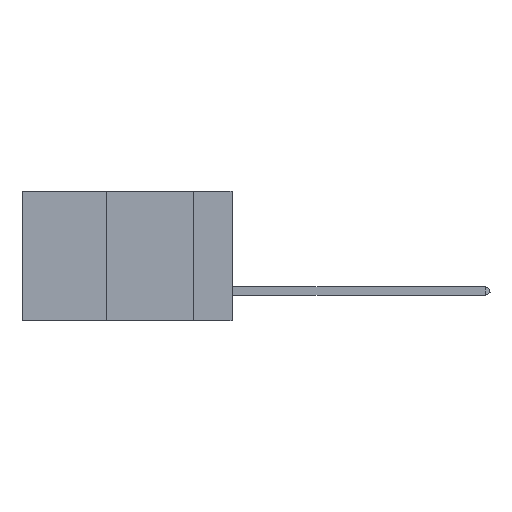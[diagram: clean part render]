
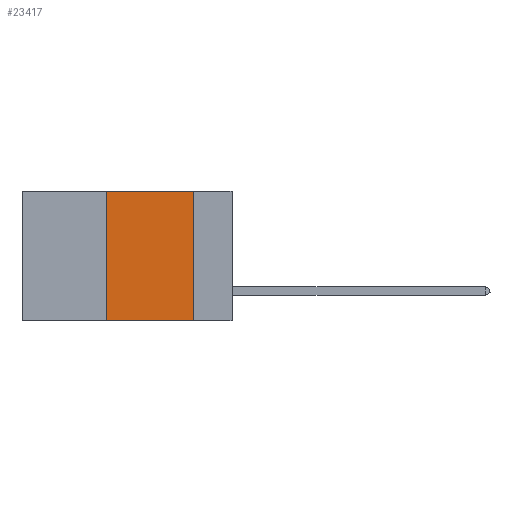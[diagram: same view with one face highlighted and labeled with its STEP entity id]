
A CAD part, left-side view. The second image highlights one B-rep face of the part: STEP entity #23417.
In plain terms, the highlighted planar face has unit normal (-1, 0, 0).
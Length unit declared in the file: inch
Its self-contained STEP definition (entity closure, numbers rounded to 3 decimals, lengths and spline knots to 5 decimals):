
#2882 = ORIENTED_EDGE ( 'NONE', *, *, #22673, .F. ) ;
#3246 = CARTESIAN_POINT ( 'NONE',  ( 0., 0.36, 0. ) ) ;
#4315 = LINE ( 'NONE', #11277, #26210 ) ;
#4737 = ORIENTED_EDGE ( 'NONE', *, *, #27943, .T. ) ;
#5513 = EDGE_CURVE ( 'NONE', #7161, #22218, #30814, .T. ) ;
#6093 = DIRECTION ( 'NONE',  ( 0., -1., 0. ) ) ;
#6734 = CARTESIAN_POINT ( 'NONE',  ( 0., 0.6, 0. ) ) ;
#7047 = ORIENTED_EDGE ( 'NONE', *, *, #29732, .F. ) ;
#7161 = VERTEX_POINT ( 'NONE', #10127 ) ;
#7401 = DIRECTION ( 'NONE',  ( 0., -1., 0. ) ) ;
#8808 = PLANE ( 'NONE',  #25609 ) ;
#10127 = CARTESIAN_POINT ( 'NONE',  ( 0., 0.36, 0. ) ) ;
#11152 = VECTOR ( 'NONE', #6093, 39.37008 ) ;
#11186 = VECTOR ( 'NONE', #7401, 39.37008 ) ;
#11277 = CARTESIAN_POINT ( 'NONE',  ( 0., 0.11, 0. ) ) ;
#11842 = VERTEX_POINT ( 'NONE', #31393 ) ;
#12524 = CARTESIAN_POINT ( 'NONE',  ( 0., 0.6, -0.37 ) ) ;
#14670 = CARTESIAN_POINT ( 'NONE',  ( 0., 0.11, -0.37 ) ) ;
#15734 = FACE_OUTER_BOUND ( 'NONE', #24932, .T. ) ;
#18116 = LINE ( 'NONE', #12524, #11186 ) ;
#20738 = DIRECTION ( 'NONE',  ( 1., 0., 0. ) ) ;
#20935 = DIRECTION ( 'NONE',  ( 0., 0., -1. ) ) ;
#21161 = CARTESIAN_POINT ( 'NONE',  ( 0., 0.6, 0. ) ) ;
#21853 = VERTEX_POINT ( 'NONE', #14670 ) ;
#22218 = VERTEX_POINT ( 'NONE', #28332 ) ;
#22450 = DIRECTION ( 'NONE',  ( 0., 0., 1. ) ) ;
#22673 = EDGE_CURVE ( 'NONE', #22218, #21853, #4315, .T. ) ;
#23417 = ADVANCED_FACE ( 'NONE', ( #15734 ), #8808, .F. ) ;
#24184 = ORIENTED_EDGE ( 'NONE', *, *, #5513, .F. ) ;
#24932 = EDGE_LOOP ( 'NONE', ( #2882, #24184, #7047, #4737 ) ) ;
#25609 = AXIS2_PLACEMENT_3D ( 'NONE', #21161, #20738, #20935 ) ;
#26210 = VECTOR ( 'NONE', #28505, 39.37008 ) ;
#26446 = LINE ( 'NONE', #3246, #29529 ) ;
#27943 = EDGE_CURVE ( 'NONE', #11842, #21853, #18116, .T. ) ;
#28332 = CARTESIAN_POINT ( 'NONE',  ( 0., 0.11, 0. ) ) ;
#28505 = DIRECTION ( 'NONE',  ( 0., 0., -1. ) ) ;
#29529 = VECTOR ( 'NONE', #22450, 39.37008 ) ;
#29732 = EDGE_CURVE ( 'NONE', #11842, #7161, #26446, .T. ) ;
#30814 = LINE ( 'NONE', #6734, #11152 ) ;
#31393 = CARTESIAN_POINT ( 'NONE',  ( 0., 0.36, -0.37 ) ) ;
